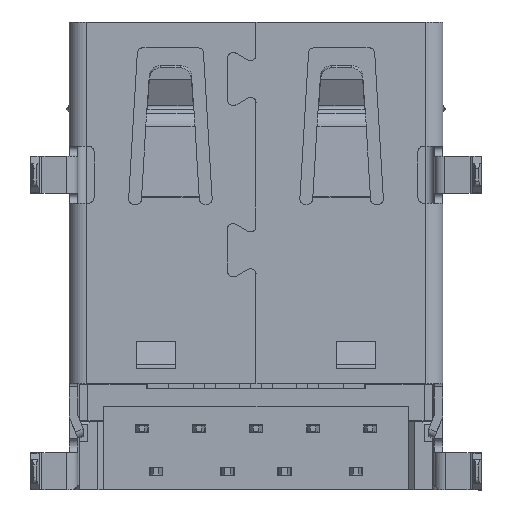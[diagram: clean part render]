
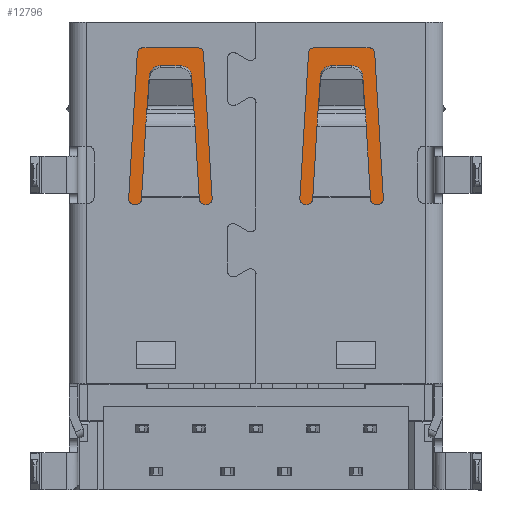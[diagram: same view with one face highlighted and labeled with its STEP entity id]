
A CAD part, front view. The second image highlights one B-rep face of the part: STEP entity #12796.
In plain terms, the highlighted planar face has unit normal (0, -1, 0).
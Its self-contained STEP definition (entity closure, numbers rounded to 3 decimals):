
#5151 = CARTESIAN_POINT ( 'NONE',  ( 3.933, 1.335, -6.924 ) ) ;
#8879 = CARTESIAN_POINT ( 'NONE',  ( -6.084, 1.335, -6.739 ) ) ;
#9074 = ORIENTED_EDGE ( 'NONE', *, *, #22656, .F. ) ;
#12146 = DIRECTION ( 'NONE',  ( -1., 0., 0. ) ) ;
#12796 = ADVANCED_FACE ( 'NONE', ( #14619 ), #37927, .F. ) ;
#14619 = FACE_OUTER_BOUND ( 'NONE', #60659, .T. ) ;
#15895 = LINE ( 'NONE', #56357, #22600 ) ;
#16659 = LINE ( 'NONE', #51771, #39290 ) ;
#19799 = CARTESIAN_POINT ( 'NONE',  ( -5.887, 1.335, -16.166 ) ) ;
#20448 = EDGE_CURVE ( 'NONE', #49072, #22613, #16659, .T. ) ;
#22600 = VECTOR ( 'NONE', #27371, 1000. ) ;
#22613 = VERTEX_POINT ( 'NONE', #5151 ) ;
#22656 = EDGE_CURVE ( 'NONE', #61889, #49072, #15895, .T. ) ;
#23579 = EDGE_CURVE ( 'NONE', #66181, #61889, #53758, .T. ) ;
#25037 = DIRECTION ( 'NONE',  ( 0., 0., -1. ) ) ;
#25327 = DIRECTION ( 'NONE',  ( 1., 0., 0. ) ) ;
#27371 = DIRECTION ( 'NONE',  ( 0., 0., 1. ) ) ;
#32194 = DIRECTION ( 'NONE',  ( 0., 1., 0. ) ) ;
#35743 = CARTESIAN_POINT ( 'NONE',  ( 3.933, 1.335, -11.545 ) ) ;
#37283 = ORIENTED_EDGE ( 'NONE', *, *, #23579, .F. ) ;
#37927 = PLANE ( 'NONE',  #42809 ) ;
#38364 = CARTESIAN_POINT ( 'NONE',  ( 3.933, 1.335, -16.166 ) ) ;
#38834 = DIRECTION ( 'NONE',  ( 1., 0., 0. ) ) ;
#39290 = VECTOR ( 'NONE', #38834, 1000. ) ;
#41177 = ORIENTED_EDGE ( 'NONE', *, *, #45077, .F. ) ;
#42217 = VECTOR ( 'NONE', #12146, 1000. ) ;
#42809 = AXIS2_PLACEMENT_3D ( 'NONE', #8879, #32194, #25327 ) ;
#45077 = EDGE_CURVE ( 'NONE', #22613, #66181, #48680, .T. ) ;
#48680 = LINE ( 'NONE', #35743, #58844 ) ;
#49072 = VERTEX_POINT ( 'NONE', #75399 ) ;
#51771 = CARTESIAN_POINT ( 'NONE',  ( -0.977, 1.335, -6.924 ) ) ;
#53758 = LINE ( 'NONE', #71265, #42217 ) ;
#56357 = CARTESIAN_POINT ( 'NONE',  ( -5.887, 1.335, -11.545 ) ) ;
#58844 = VECTOR ( 'NONE', #25037, 1000. ) ;
#60659 = EDGE_LOOP ( 'NONE', ( #9074, #37283, #41177, #64441 ) ) ;
#61889 = VERTEX_POINT ( 'NONE', #19799 ) ;
#64441 = ORIENTED_EDGE ( 'NONE', *, *, #20448, .F. ) ;
#66181 = VERTEX_POINT ( 'NONE', #38364 ) ;
#71265 = CARTESIAN_POINT ( 'NONE',  ( -0.977, 1.335, -16.166 ) ) ;
#75399 = CARTESIAN_POINT ( 'NONE',  ( -5.887, 1.335, -6.924 ) ) ;
